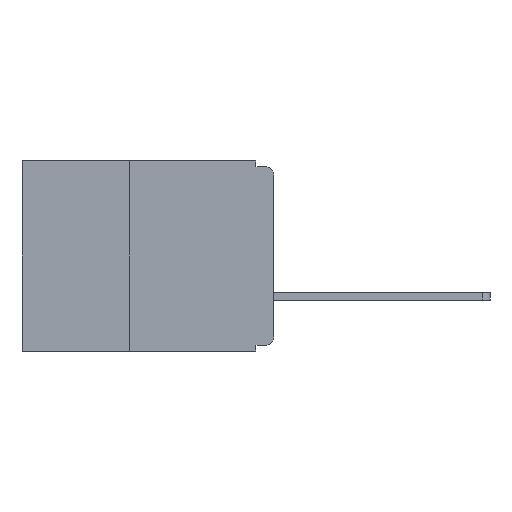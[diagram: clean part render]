
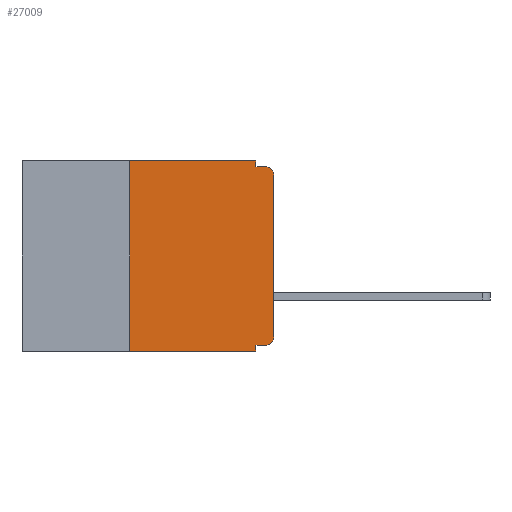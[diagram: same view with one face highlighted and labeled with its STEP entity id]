
A CAD part, left-side view. The second image highlights one B-rep face of the part: STEP entity #27009.
In plain terms, the highlighted planar face has unit normal (-1, 0, 0).
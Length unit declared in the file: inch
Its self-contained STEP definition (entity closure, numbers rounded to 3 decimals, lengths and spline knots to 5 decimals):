
#115 = EDGE_CURVE ( 'NONE', #22212, #16936, #25595, .T. ) ;
#169 = CARTESIAN_POINT ( 'NONE',  ( 0., 0.031, -0.33 ) ) ;
#370 = VECTOR ( 'NONE', #7145, 39.37008 ) ;
#1772 = LINE ( 'NONE', #11030, #12460 ) ;
#2050 = EDGE_CURVE ( 'NONE', #22242, #10054, #17374, .T. ) ;
#2221 = CARTESIAN_POINT ( 'NONE',  ( 0., 0.031, -0.01 ) ) ;
#3235 = ORIENTED_EDGE ( 'NONE', *, *, #2050, .F. ) ;
#3571 = VECTOR ( 'NONE', #16613, 39.37008 ) ;
#4086 = PLANE ( 'NONE',  #14189 ) ;
#4173 = DIRECTION ( 'NONE',  ( 1., 0., 0. ) ) ;
#4370 = ORIENTED_EDGE ( 'NONE', *, *, #26647, .F. ) ;
#4763 = EDGE_LOOP ( 'NONE', ( #13714, #16392, #4370, #14573, #5136, #7808, #22236, #3235, #10432, #18759 ) ) ;
#5136 = ORIENTED_EDGE ( 'NONE', *, *, #17983, .F. ) ;
#5139 = EDGE_CURVE ( 'NONE', #23794, #22242, #18240, .T. ) ;
#5976 = VECTOR ( 'NONE', #23294, 39.37008 ) ;
#6704 = CARTESIAN_POINT ( 'NONE',  ( 0., 0.25, -0.33 ) ) ;
#6826 = VECTOR ( 'NONE', #9826, 39.37008 ) ;
#7145 = DIRECTION ( 'NONE',  ( 0., -1., 0. ) ) ;
#7213 = EDGE_CURVE ( 'NONE', #26993, #22736, #1772, .T. ) ;
#7309 = FACE_OUTER_BOUND ( 'NONE', #4763, .T. ) ;
#7366 = VERTEX_POINT ( 'NONE', #24370 ) ;
#7758 = CARTESIAN_POINT ( 'NONE',  ( 0., 0.015, -0.32 ) ) ;
#7808 = ORIENTED_EDGE ( 'NONE', *, *, #115, .F. ) ;
#9113 = DIRECTION ( 'NONE',  ( -1., 0., 0. ) ) ;
#9756 = VERTEX_POINT ( 'NONE', #16123 ) ;
#9826 = DIRECTION ( 'NONE',  ( 0., 1., 0. ) ) ;
#10054 = VERTEX_POINT ( 'NONE', #169 ) ;
#10391 = CARTESIAN_POINT ( 'NONE',  ( 0., 0.015, -0.305 ) ) ;
#10432 = ORIENTED_EDGE ( 'NONE', *, *, #5139, .F. ) ;
#10714 = VECTOR ( 'NONE', #27591, 39.37008 ) ;
#11030 = CARTESIAN_POINT ( 'NONE',  ( 0., 0.031, 0. ) ) ;
#11379 = LINE ( 'NONE', #14777, #10714 ) ;
#11427 = EDGE_CURVE ( 'NONE', #23794, #16388, #15245, .T. ) ;
#12460 = VECTOR ( 'NONE', #13155, 39.37008 ) ;
#12525 = DIRECTION ( 'NONE',  ( 0., 0., -1. ) ) ;
#13155 = DIRECTION ( 'NONE',  ( 0., 0., -1. ) ) ;
#13161 = CARTESIAN_POINT ( 'NONE',  ( 0., 0.031, -0.32 ) ) ;
#13714 = ORIENTED_EDGE ( 'NONE', *, *, #15531, .T. ) ;
#14189 = AXIS2_PLACEMENT_3D ( 'NONE', #16980, #4173, #19144 ) ;
#14454 = CARTESIAN_POINT ( 'NONE',  ( 0., 0.437, 0. ) ) ;
#14573 = ORIENTED_EDGE ( 'NONE', *, *, #7213, .F. ) ;
#14777 = CARTESIAN_POINT ( 'NONE',  ( 0., 0., 0. ) ) ;
#14829 = CARTESIAN_POINT ( 'NONE',  ( 0., 0.031, 0. ) ) ;
#14944 = EDGE_CURVE ( 'NONE', #22212, #10054, #26786, .T. ) ;
#14992 = DIRECTION ( 'NONE',  ( 0., -1., 0. ) ) ;
#15245 = CIRCLE ( 'NONE', #27196, 0.015 ) ;
#15531 = EDGE_CURVE ( 'NONE', #16388, #9756, #11379, .T. ) ;
#15728 = CARTESIAN_POINT ( 'NONE',  ( 0., 0., -0.305 ) ) ;
#15902 = CARTESIAN_POINT ( 'NONE',  ( 0., 0.031, -0.33 ) ) ;
#16123 = CARTESIAN_POINT ( 'NONE',  ( 0., 0., -0.025 ) ) ;
#16388 = VERTEX_POINT ( 'NONE', #15728 ) ;
#16392 = ORIENTED_EDGE ( 'NONE', *, *, #22881, .T. ) ;
#16613 = DIRECTION ( 'NONE',  ( 0., -1., 0. ) ) ;
#16936 = VERTEX_POINT ( 'NONE', #23929 ) ;
#16980 = CARTESIAN_POINT ( 'NONE',  ( 0., 0.437, 0. ) ) ;
#17342 = CIRCLE ( 'NONE', #26502, 0.015 ) ;
#17374 = LINE ( 'NONE', #15902, #5976 ) ;
#17983 = EDGE_CURVE ( 'NONE', #16936, #26993, #26985, .T. ) ;
#18240 = LINE ( 'NONE', #24775, #6826 ) ;
#18759 = ORIENTED_EDGE ( 'NONE', *, *, #11427, .T. ) ;
#19144 = DIRECTION ( 'NONE',  ( 0., 0., -1. ) ) ;
#19202 = CARTESIAN_POINT ( 'NONE',  ( 0., 0.437, -0.33 ) ) ;
#20764 = CARTESIAN_POINT ( 'NONE',  ( 0., 0.25, -0.33 ) ) ;
#21716 = LINE ( 'NONE', #22099, #370 ) ;
#21895 = CARTESIAN_POINT ( 'NONE',  ( 0., 0.015, -0.025 ) ) ;
#22099 = CARTESIAN_POINT ( 'NONE',  ( 0., 0., -0.01 ) ) ;
#22212 = VERTEX_POINT ( 'NONE', #6704 ) ;
#22236 = ORIENTED_EDGE ( 'NONE', *, *, #14944, .T. ) ;
#22242 = VERTEX_POINT ( 'NONE', #13161 ) ;
#22736 = VERTEX_POINT ( 'NONE', #2221 ) ;
#22881 = EDGE_CURVE ( 'NONE', #9756, #7366, #17342, .T. ) ;
#23294 = DIRECTION ( 'NONE',  ( 0., 0., -1. ) ) ;
#23794 = VERTEX_POINT ( 'NONE', #7758 ) ;
#23929 = CARTESIAN_POINT ( 'NONE',  ( 0., 0.25, 0. ) ) ;
#24070 = DIRECTION ( 'NONE',  ( 0., 0., -1. ) ) ;
#24370 = CARTESIAN_POINT ( 'NONE',  ( 0., 0.015, -0.01 ) ) ;
#24775 = CARTESIAN_POINT ( 'NONE',  ( 0., 0., -0.32 ) ) ;
#24895 = VECTOR ( 'NONE', #26849, 39.37008 ) ;
#25341 = DIRECTION ( 'NONE',  ( -1., 0., 0. ) ) ;
#25595 = LINE ( 'NONE', #20764, #24895 ) ;
#26125 = VECTOR ( 'NONE', #14992, 39.37008 ) ;
#26502 = AXIS2_PLACEMENT_3D ( 'NONE', #21895, #9113, #24070 ) ;
#26647 = EDGE_CURVE ( 'NONE', #22736, #7366, #21716, .T. ) ;
#26786 = LINE ( 'NONE', #19202, #26125 ) ;
#26849 = DIRECTION ( 'NONE',  ( 0., 0., 1. ) ) ;
#26985 = LINE ( 'NONE', #14454, #3571 ) ;
#26993 = VERTEX_POINT ( 'NONE', #14829 ) ;
#27009 = ADVANCED_FACE ( 'NONE', ( #7309 ), #4086, .F. ) ;
#27196 = AXIS2_PLACEMENT_3D ( 'NONE', #10391, #25341, #12525 ) ;
#27591 = DIRECTION ( 'NONE',  ( 0., 0., 1. ) ) ;
